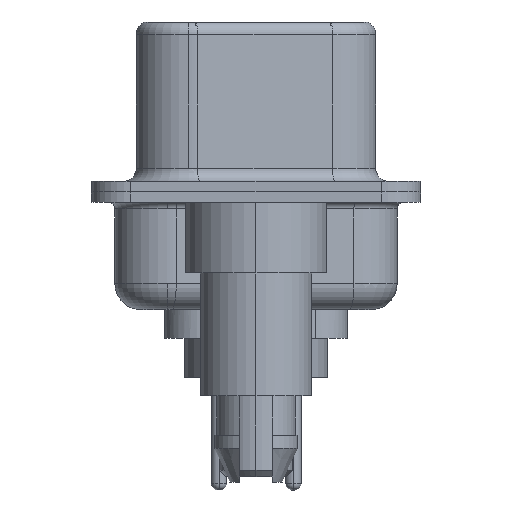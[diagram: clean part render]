
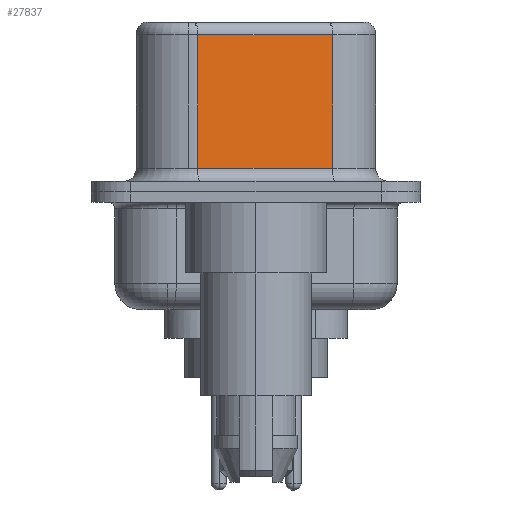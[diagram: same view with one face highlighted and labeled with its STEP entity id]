
A CAD part, left-side view. The second image highlights one B-rep face of the part: STEP entity #27837.
In plain terms, the highlighted planar face has unit normal (-0.985, -0.174, 0).
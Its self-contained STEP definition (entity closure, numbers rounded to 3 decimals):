
#1164 = DIRECTION ( 'NONE',  ( 0.174, -0.985, 0. ) ) ;
#1516 = VECTOR ( 'NONE', #5247, 1000. ) ;
#1687 = VECTOR ( 'NONE', #1164, 1000. ) ;
#2408 = LINE ( 'NONE', #25141, #1687 ) ;
#4326 = VERTEX_POINT ( 'NONE', #15193 ) ;
#4941 = CARTESIAN_POINT ( 'NONE',  ( 4.58, -2.927, 0.9 ) ) ;
#5247 = DIRECTION ( 'NONE',  ( 0., 0., -1. ) ) ;
#5515 = VECTOR ( 'NONE', #7005, 1000. ) ;
#6566 = DIRECTION ( 'NONE',  ( 0.985, 0.174, 0. ) ) ;
#6706 = VERTEX_POINT ( 'NONE', #4941 ) ;
#7005 = DIRECTION ( 'NONE',  ( 0., 0., -1. ) ) ;
#7432 = LINE ( 'NONE', #18258, #1516 ) ;
#8718 = VERTEX_POINT ( 'NONE', #12114 ) ;
#9386 = EDGE_CURVE ( 'NONE', #23272, #6706, #2408, .T. ) ;
#9998 = AXIS2_PLACEMENT_3D ( 'NONE', #19582, #6566, #21750 ) ;
#11194 = EDGE_CURVE ( 'NONE', #4326, #8718, #15818, .T. ) ;
#12114 = CARTESIAN_POINT ( 'NONE',  ( 3.67, 2.233, 6.02 ) ) ;
#12721 = EDGE_LOOP ( 'NONE', ( #24481, #21497, #14448, #23903 ) ) ;
#14448 = ORIENTED_EDGE ( 'NONE', *, *, #21105, .T. ) ;
#15193 = CARTESIAN_POINT ( 'NONE',  ( 4.58, -2.927, 6.02 ) ) ;
#15796 = CARTESIAN_POINT ( 'NONE',  ( 3.67, 2.233, 0.9 ) ) ;
#15818 = LINE ( 'NONE', #25642, #20891 ) ;
#16628 = FACE_OUTER_BOUND ( 'NONE', #12721, .T. ) ;
#18258 = CARTESIAN_POINT ( 'NONE',  ( 3.67, 2.233, 6.52 ) ) ;
#19582 = CARTESIAN_POINT ( 'NONE',  ( 4.58, -2.927, 6.52 ) ) ;
#20018 = CARTESIAN_POINT ( 'NONE',  ( 4.58, -2.927, 6.52 ) ) ;
#20891 = VECTOR ( 'NONE', #27864, 1000. ) ;
#21105 = EDGE_CURVE ( 'NONE', #8718, #23272, #7432, .T. ) ;
#21497 = ORIENTED_EDGE ( 'NONE', *, *, #11194, .T. ) ;
#21750 = DIRECTION ( 'NONE',  ( -0.174, 0.985, 0. ) ) ;
#22822 = LINE ( 'NONE', #20018, #5515 ) ;
#23272 = VERTEX_POINT ( 'NONE', #15796 ) ;
#23666 = PLANE ( 'NONE',  #9998 ) ;
#23903 = ORIENTED_EDGE ( 'NONE', *, *, #9386, .T. ) ;
#24481 = ORIENTED_EDGE ( 'NONE', *, *, #25339, .F. ) ;
#25141 = CARTESIAN_POINT ( 'NONE',  ( 4.58, -2.927, 0.9 ) ) ;
#25339 = EDGE_CURVE ( 'NONE', #4326, #6706, #22822, .T. ) ;
#25642 = CARTESIAN_POINT ( 'NONE',  ( 4.58, -2.927, 6.02 ) ) ;
#27837 = ADVANCED_FACE ( 'NONE', ( #16628 ), #23666, .F. ) ;
#27864 = DIRECTION ( 'NONE',  ( -0.174, 0.985, 0. ) ) ;
